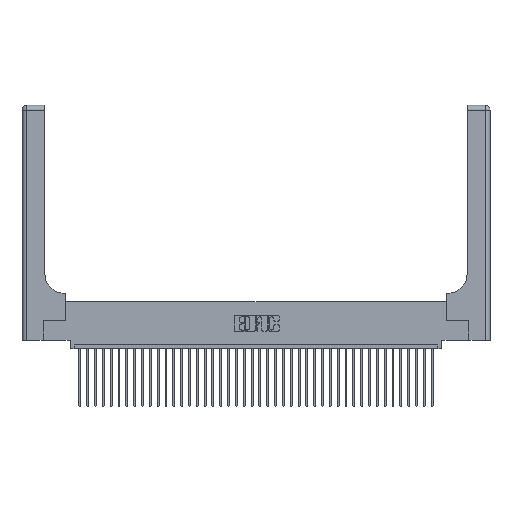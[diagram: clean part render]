
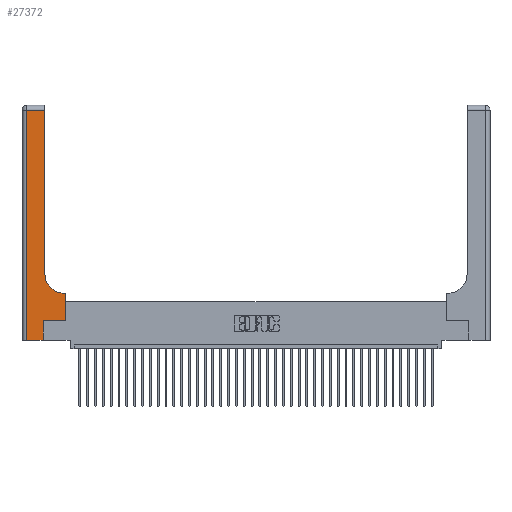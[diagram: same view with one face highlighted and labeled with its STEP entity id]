
A CAD part, top view. The second image highlights one B-rep face of the part: STEP entity #27372.
In plain terms, the highlighted planar face has unit normal (0, 0, 1).
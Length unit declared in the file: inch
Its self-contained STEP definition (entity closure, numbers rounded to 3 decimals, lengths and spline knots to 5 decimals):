
#370 = LINE ( 'NONE', #903, #825 ) ;
#825 = VECTOR ( 'NONE', #31375, 39.37008 ) ;
#903 = CARTESIAN_POINT ( 'NONE',  ( 0.06, 3., 0.37 ) ) ;
#1664 = VECTOR ( 'NONE', #34754, 39.37008 ) ;
#2125 = DIRECTION ( 'NONE',  ( 0., 0., -1. ) ) ;
#2323 = ORIENTED_EDGE ( 'NONE', *, *, #23196, .T. ) ;
#3004 = CARTESIAN_POINT ( 'NONE',  ( 0.2915, 3., 0.37 ) ) ;
#6233 = VERTEX_POINT ( 'NONE', #34273 ) ;
#6583 = VERTEX_POINT ( 'NONE', #18541 ) ;
#8098 = AXIS2_PLACEMENT_3D ( 'NONE', #23417, #2125, #34999 ) ;
#8103 = PLANE ( 'NONE',  #8098 ) ;
#8471 = EDGE_CURVE ( 'NONE', #27894, #33717, #37211, .T. ) ;
#8794 = LINE ( 'NONE', #32364, #1664 ) ;
#9861 = CARTESIAN_POINT ( 'NONE',  ( 0.269, 0.25, 0.37 ) ) ;
#12179 = VERTEX_POINT ( 'NONE', #35765 ) ;
#13006 = CARTESIAN_POINT ( 'NONE',  ( 0.06, 2.94, 0.37 ) ) ;
#13103 = LINE ( 'NONE', #29126, #36458 ) ;
#13411 = DIRECTION ( 'NONE',  ( 1., 0., 0. ) ) ;
#13598 = FACE_OUTER_BOUND ( 'NONE', #22198, .T. ) ;
#14502 = EDGE_CURVE ( 'NONE', #6583, #32198, #30594, .T. ) ;
#15386 = VECTOR ( 'NONE', #29908, 39.37008 ) ;
#15429 = ORIENTED_EDGE ( 'NONE', *, *, #38162, .T. ) ;
#16455 = AXIS2_PLACEMENT_3D ( 'NONE', #24254, #18059, #30373 ) ;
#17487 = VECTOR ( 'NONE', #23741, 39.37008 ) ;
#18059 = DIRECTION ( 'NONE',  ( 0., 0., -1. ) ) ;
#18212 = VERTEX_POINT ( 'NONE', #34719 ) ;
#18541 = CARTESIAN_POINT ( 'NONE',  ( 0.2915, 0.85, 0.37 ) ) ;
#18558 = CIRCLE ( 'NONE', #16455, 0.25 ) ;
#18719 = VECTOR ( 'NONE', #22257, 39.37008 ) ;
#19376 = DIRECTION ( 'NONE',  ( 0., 1., 0. ) ) ;
#19553 = CARTESIAN_POINT ( 'NONE',  ( 0., 0., 0.37 ) ) ;
#19681 = LINE ( 'NONE', #34375, #18719 ) ;
#19711 = VERTEX_POINT ( 'NONE', #13006 ) ;
#20551 = EDGE_CURVE ( 'NONE', #19711, #27894, #370, .T. ) ;
#21652 = ORIENTED_EDGE ( 'NONE', *, *, #8471, .T. ) ;
#21709 = LINE ( 'NONE', #32681, #17487 ) ;
#21955 = EDGE_CURVE ( 'NONE', #32198, #19711, #13103, .T. ) ;
#22198 = EDGE_LOOP ( 'NONE', ( #27186, #33210, #26732, #21652, #34178, #2323, #15429, #22661, #39072 ) ) ;
#22257 = DIRECTION ( 'NONE',  ( -1., 0., 0. ) ) ;
#22661 = ORIENTED_EDGE ( 'NONE', *, *, #28519, .T. ) ;
#23196 = EDGE_CURVE ( 'NONE', #28442, #6233, #8794, .T. ) ;
#23417 = CARTESIAN_POINT ( 'NONE',  ( 0., 3., 0.37 ) ) ;
#23741 = DIRECTION ( 'NONE',  ( 0., 1., 0. ) ) ;
#24254 = CARTESIAN_POINT ( 'NONE',  ( 0.5415, 0.85, 0.37 ) ) ;
#24371 = EDGE_CURVE ( 'NONE', #12179, #6583, #18558, .T. ) ;
#25272 = CARTESIAN_POINT ( 'NONE',  ( 0.269, 0., 0.37 ) ) ;
#25334 = CARTESIAN_POINT ( 'NONE',  ( 0.5585, 0.25, 0.37 ) ) ;
#26732 = ORIENTED_EDGE ( 'NONE', *, *, #20551, .T. ) ;
#26909 = CARTESIAN_POINT ( 'NONE',  ( 0.2915, 2.94, 0.37 ) ) ;
#27186 = ORIENTED_EDGE ( 'NONE', *, *, #14502, .T. ) ;
#27372 = ADVANCED_FACE ( 'NONE', ( #13598 ), #8103, .F. ) ;
#27894 = VERTEX_POINT ( 'NONE', #28539 ) ;
#28442 = VERTEX_POINT ( 'NONE', #9861 ) ;
#28519 = EDGE_CURVE ( 'NONE', #18212, #12179, #19681, .T. ) ;
#28539 = CARTESIAN_POINT ( 'NONE',  ( 0.06, 0., 0.37 ) ) ;
#29126 = CARTESIAN_POINT ( 'NONE',  ( 0., 2.94, 0.37 ) ) ;
#29378 = DIRECTION ( 'NONE',  ( -1., 0., 0. ) ) ;
#29908 = DIRECTION ( 'NONE',  ( 0., 1., 0. ) ) ;
#30373 = DIRECTION ( 'NONE',  ( 1., 0., 0. ) ) ;
#30594 = LINE ( 'NONE', #3004, #15386 ) ;
#31375 = DIRECTION ( 'NONE',  ( 0., -1., 0. ) ) ;
#32198 = VERTEX_POINT ( 'NONE', #26909 ) ;
#32364 = CARTESIAN_POINT ( 'NONE',  ( 0.269, 0.25, 0.37 ) ) ;
#32681 = CARTESIAN_POINT ( 'NONE',  ( 0.269, 0., 0.37 ) ) ;
#33210 = ORIENTED_EDGE ( 'NONE', *, *, #21955, .T. ) ;
#33491 = EDGE_CURVE ( 'NONE', #33717, #28442, #21709, .T. ) ;
#33717 = VERTEX_POINT ( 'NONE', #25272 ) ;
#34178 = ORIENTED_EDGE ( 'NONE', *, *, #33491, .T. ) ;
#34273 = CARTESIAN_POINT ( 'NONE',  ( 0.5585, 0.25, 0.37 ) ) ;
#34375 = CARTESIAN_POINT ( 'NONE',  ( 0.2915, 0.6, 0.37 ) ) ;
#34719 = CARTESIAN_POINT ( 'NONE',  ( 0.5585, 0.6, 0.37 ) ) ;
#34754 = DIRECTION ( 'NONE',  ( 1., 0., 0. ) ) ;
#34999 = DIRECTION ( 'NONE',  ( -1., 0., 0. ) ) ;
#35765 = CARTESIAN_POINT ( 'NONE',  ( 0.5415, 0.6, 0.37 ) ) ;
#36291 = VECTOR ( 'NONE', #13411, 39.37008 ) ;
#36458 = VECTOR ( 'NONE', #29378, 39.37008 ) ;
#36894 = VECTOR ( 'NONE', #19376, 39.37008 ) ;
#37211 = LINE ( 'NONE', #19553, #36291 ) ;
#38162 = EDGE_CURVE ( 'NONE', #6233, #18212, #38813, .T. ) ;
#38813 = LINE ( 'NONE', #25334, #36894 ) ;
#39072 = ORIENTED_EDGE ( 'NONE', *, *, #24371, .T. ) ;
